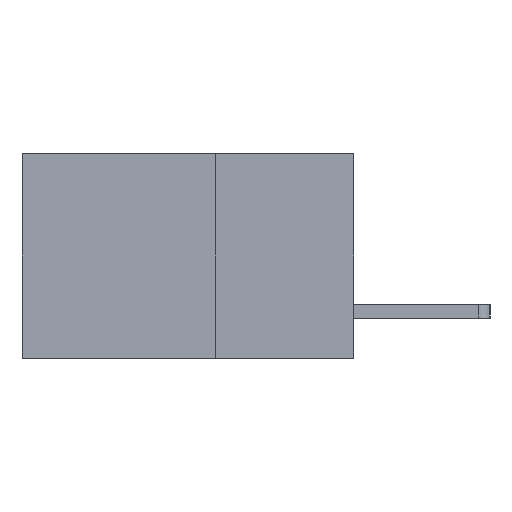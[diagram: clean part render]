
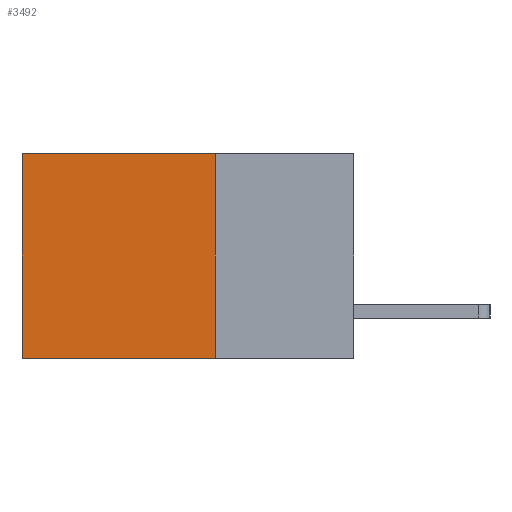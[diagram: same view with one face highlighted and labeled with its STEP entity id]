
A CAD part, left-side view. The second image highlights one B-rep face of the part: STEP entity #3492.
In plain terms, the highlighted planar face has unit normal (-1, 0, 0).
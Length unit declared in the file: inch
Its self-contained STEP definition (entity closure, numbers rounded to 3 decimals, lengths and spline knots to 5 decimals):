
#512 = VERTEX_POINT ( 'NONE', #10633 ) ;
#707 = CARTESIAN_POINT ( 'NONE',  ( 0.2875, 0.6, -0.37 ) ) ;
#1074 = PLANE ( 'NONE',  #4968 ) ;
#2099 = FACE_OUTER_BOUND ( 'NONE', #6138, .T. ) ;
#2211 = CARTESIAN_POINT ( 'NONE',  ( 0.2875, 0.25, -0.37 ) ) ;
#2282 = DIRECTION ( 'NONE',  ( 1., 0., 0. ) ) ;
#2485 = CARTESIAN_POINT ( 'NONE',  ( 0.2875, 0.25, 0. ) ) ;
#2601 = CARTESIAN_POINT ( 'NONE',  ( 0.2875, 0.6, 0. ) ) ;
#2705 = CARTESIAN_POINT ( 'NONE',  ( 0.2875, 0.25, 0. ) ) ;
#2929 = VECTOR ( 'NONE', #7702, 39.37008 ) ;
#3155 = VECTOR ( 'NONE', #4569, 39.37008 ) ;
#3492 = ADVANCED_FACE ( 'NONE', ( #2099 ), #1074, .F. ) ;
#3624 = VECTOR ( 'NONE', #7241, 39.37008 ) ;
#4006 = LINE ( 'NONE', #6969, #3624 ) ;
#4093 = DIRECTION ( 'NONE',  ( 0., 0., -1. ) ) ;
#4569 = DIRECTION ( 'NONE',  ( 0., 0., -1. ) ) ;
#4823 = EDGE_CURVE ( 'NONE', #10610, #7764, #12679, .T. ) ;
#4968 = AXIS2_PLACEMENT_3D ( 'NONE', #8437, #2282, #4093 ) ;
#6138 = EDGE_LOOP ( 'NONE', ( #11381, #9789, #11873, #7558 ) ) ;
#6237 = VERTEX_POINT ( 'NONE', #2485 ) ;
#6374 = EDGE_CURVE ( 'NONE', #6237, #10610, #4006, .T. ) ;
#6397 = DIRECTION ( 'NONE',  ( 0., 1., 0. ) ) ;
#6969 = CARTESIAN_POINT ( 'NONE',  ( 0.2875, 0.25, 0. ) ) ;
#7241 = DIRECTION ( 'NONE',  ( 0., 1., 0. ) ) ;
#7314 = CARTESIAN_POINT ( 'NONE',  ( 0.2875, 0.6, 0. ) ) ;
#7558 = ORIENTED_EDGE ( 'NONE', *, *, #6374, .T. ) ;
#7702 = DIRECTION ( 'NONE',  ( 0., 0., -1. ) ) ;
#7764 = VERTEX_POINT ( 'NONE', #707 ) ;
#7887 = LINE ( 'NONE', #2705, #3155 ) ;
#8437 = CARTESIAN_POINT ( 'NONE',  ( 0.2875, 0.25, 0. ) ) ;
#8550 = EDGE_CURVE ( 'NONE', #512, #7764, #9591, .T. ) ;
#9487 = EDGE_CURVE ( 'NONE', #6237, #512, #7887, .T. ) ;
#9591 = LINE ( 'NONE', #2211, #11735 ) ;
#9789 = ORIENTED_EDGE ( 'NONE', *, *, #8550, .F. ) ;
#10610 = VERTEX_POINT ( 'NONE', #2601 ) ;
#10633 = CARTESIAN_POINT ( 'NONE',  ( 0.2875, 0.25, -0.37 ) ) ;
#11381 = ORIENTED_EDGE ( 'NONE', *, *, #4823, .T. ) ;
#11735 = VECTOR ( 'NONE', #6397, 39.37008 ) ;
#11873 = ORIENTED_EDGE ( 'NONE', *, *, #9487, .F. ) ;
#12679 = LINE ( 'NONE', #7314, #2929 ) ;
